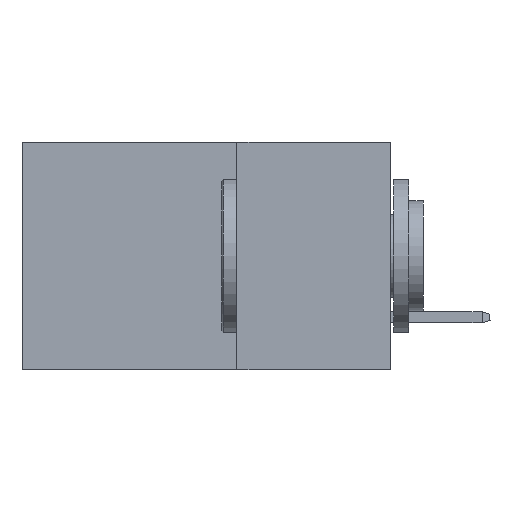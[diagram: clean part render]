
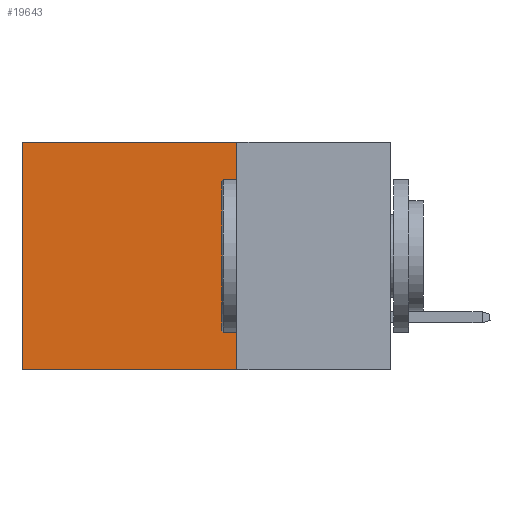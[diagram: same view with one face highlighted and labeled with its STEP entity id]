
A CAD part, left-side view. The second image highlights one B-rep face of the part: STEP entity #19643.
In plain terms, the highlighted planar face has unit normal (-1, 0, 0).
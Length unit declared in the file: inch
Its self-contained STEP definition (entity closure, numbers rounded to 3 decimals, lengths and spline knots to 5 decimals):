
#85 = LINE ( 'NONE', #18407, #11066 ) ;
#468 = AXIS2_PLACEMENT_3D ( 'NONE', #1117, #4382, #9682 ) ;
#1117 = CARTESIAN_POINT ( 'NONE',  ( 0.2875, 0.25, 0. ) ) ;
#1710 = VERTEX_POINT ( 'NONE', #2756 ) ;
#2520 = LINE ( 'NONE', #16749, #5068 ) ;
#2756 = CARTESIAN_POINT ( 'NONE',  ( 0.2875, 0.25, -0.37 ) ) ;
#3279 = CARTESIAN_POINT ( 'NONE',  ( 0.2875, 0.25, 0. ) ) ;
#3296 = EDGE_CURVE ( 'NONE', #1710, #6266, #7668, .T. ) ;
#3717 = ORIENTED_EDGE ( 'NONE', *, *, #5115, .T. ) ;
#4382 = DIRECTION ( 'NONE',  ( 1., 0., 0. ) ) ;
#5068 = VECTOR ( 'NONE', #12151, 39.37008 ) ;
#5115 = EDGE_CURVE ( 'NONE', #11722, #21171, #2520, .T. ) ;
#5949 = PLANE ( 'NONE',  #468 ) ;
#6266 = VERTEX_POINT ( 'NONE', #10820 ) ;
#6431 = DIRECTION ( 'NONE',  ( 0., 0., -1. ) ) ;
#6683 = DIRECTION ( 'NONE',  ( 0., 0., -1. ) ) ;
#7668 = LINE ( 'NONE', #11684, #18719 ) ;
#8383 = EDGE_CURVE ( 'NONE', #11722, #1710, #17660, .T. ) ;
#9492 = CARTESIAN_POINT ( 'NONE',  ( 0.2875, 0.25, 0. ) ) ;
#9682 = DIRECTION ( 'NONE',  ( 0., 0., -1. ) ) ;
#10018 = DIRECTION ( 'NONE',  ( 0., 1., 0. ) ) ;
#10312 = EDGE_LOOP ( 'NONE', ( #18629, #13895, #13321, #3717 ) ) ;
#10820 = CARTESIAN_POINT ( 'NONE',  ( 0.2875, 0.6, -0.37 ) ) ;
#11066 = VECTOR ( 'NONE', #6683, 39.37008 ) ;
#11684 = CARTESIAN_POINT ( 'NONE',  ( 0.2875, 0.25, -0.37 ) ) ;
#11722 = VERTEX_POINT ( 'NONE', #3279 ) ;
#12151 = DIRECTION ( 'NONE',  ( 0., 1., 0. ) ) ;
#13321 = ORIENTED_EDGE ( 'NONE', *, *, #8383, .F. ) ;
#13895 = ORIENTED_EDGE ( 'NONE', *, *, #3296, .F. ) ;
#14864 = EDGE_CURVE ( 'NONE', #21171, #6266, #85, .T. ) ;
#16749 = CARTESIAN_POINT ( 'NONE',  ( 0.2875, 0.25, 0. ) ) ;
#16759 = CARTESIAN_POINT ( 'NONE',  ( 0.2875, 0.6, 0. ) ) ;
#17660 = LINE ( 'NONE', #9492, #19217 ) ;
#18407 = CARTESIAN_POINT ( 'NONE',  ( 0.2875, 0.6, 0. ) ) ;
#18629 = ORIENTED_EDGE ( 'NONE', *, *, #14864, .T. ) ;
#18719 = VECTOR ( 'NONE', #10018, 39.37008 ) ;
#19217 = VECTOR ( 'NONE', #6431, 39.37008 ) ;
#19442 = FACE_OUTER_BOUND ( 'NONE', #10312, .T. ) ;
#19643 = ADVANCED_FACE ( 'NONE', ( #19442 ), #5949, .F. ) ;
#21171 = VERTEX_POINT ( 'NONE', #16759 ) ;
